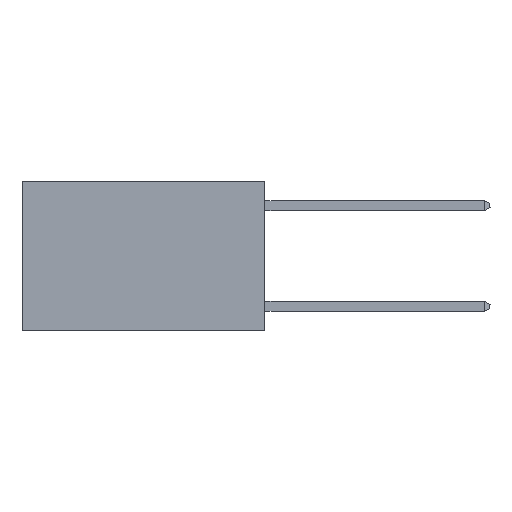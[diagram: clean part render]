
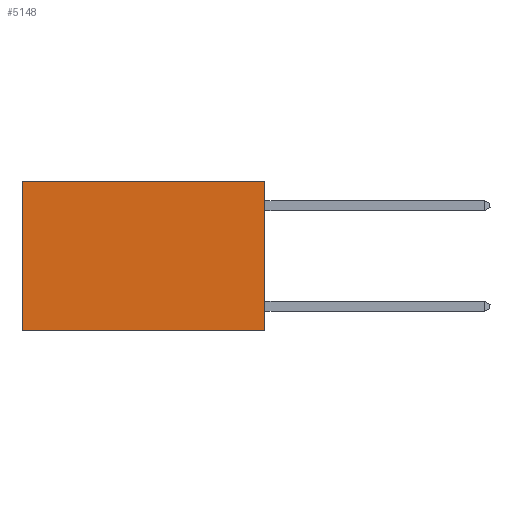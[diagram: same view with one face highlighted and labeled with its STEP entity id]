
A CAD part, left-side view. The second image highlights one B-rep face of the part: STEP entity #5148.
In plain terms, the highlighted planar face has unit normal (-1, 0, 0).
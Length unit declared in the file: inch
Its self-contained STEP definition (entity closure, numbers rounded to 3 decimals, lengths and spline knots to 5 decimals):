
#592 = VERTEX_POINT ( 'NONE', #12419 ) ;
#598 = CARTESIAN_POINT ( 'NONE',  ( 0.2625, 0., 0. ) ) ;
#2513 = ORIENTED_EDGE ( 'NONE', *, *, #7910, .F. ) ;
#3493 = VECTOR ( 'NONE', #13139, 39.37008 ) ;
#5148 = ADVANCED_FACE ( 'NONE', ( #5627 ), #16722, .F. ) ;
#5163 = ORIENTED_EDGE ( 'NONE', *, *, #24002, .T. ) ;
#5627 = FACE_OUTER_BOUND ( 'NONE', #24425, .T. ) ;
#6608 = VECTOR ( 'NONE', #28049, 39.37008 ) ;
#7044 = VERTEX_POINT ( 'NONE', #598 ) ;
#7422 = CARTESIAN_POINT ( 'NONE',  ( 0.2625, 0.6, 0. ) ) ;
#7807 = CARTESIAN_POINT ( 'NONE',  ( 0.2625, 0.6, -0.37 ) ) ;
#7910 = EDGE_CURVE ( 'NONE', #7044, #592, #19146, .T. ) ;
#8256 = DIRECTION ( 'NONE',  ( 1., 0., 0. ) ) ;
#9768 = LINE ( 'NONE', #16465, #15354 ) ;
#10593 = EDGE_CURVE ( 'NONE', #592, #24488, #26224, .T. ) ;
#12419 = CARTESIAN_POINT ( 'NONE',  ( 0.2625, 0., -0.37 ) ) ;
#13139 = DIRECTION ( 'NONE',  ( 0., 1., 0. ) ) ;
#15354 = VECTOR ( 'NONE', #27474, 39.37008 ) ;
#15512 = CARTESIAN_POINT ( 'NONE',  ( 0.2625, 0., -0.37 ) ) ;
#15884 = CARTESIAN_POINT ( 'NONE',  ( 0.2625, 0.6, 0. ) ) ;
#16465 = CARTESIAN_POINT ( 'NONE',  ( 0.2625, 0., 0. ) ) ;
#16722 = PLANE ( 'NONE',  #17514 ) ;
#17030 = EDGE_CURVE ( 'NONE', #28348, #24488, #18834, .T. ) ;
#17514 = AXIS2_PLACEMENT_3D ( 'NONE', #23709, #8256, #19095 ) ;
#18834 = LINE ( 'NONE', #7422, #6608 ) ;
#19095 = DIRECTION ( 'NONE',  ( 0., 0., -1. ) ) ;
#19146 = LINE ( 'NONE', #21529, #24289 ) ;
#21231 = DIRECTION ( 'NONE',  ( 0., 0., -1. ) ) ;
#21529 = CARTESIAN_POINT ( 'NONE',  ( 0.2625, 0., 0. ) ) ;
#23230 = ORIENTED_EDGE ( 'NONE', *, *, #17030, .T. ) ;
#23709 = CARTESIAN_POINT ( 'NONE',  ( 0.2625, 0., 0. ) ) ;
#24002 = EDGE_CURVE ( 'NONE', #7044, #28348, #9768, .T. ) ;
#24266 = ORIENTED_EDGE ( 'NONE', *, *, #10593, .F. ) ;
#24289 = VECTOR ( 'NONE', #21231, 39.37008 ) ;
#24425 = EDGE_LOOP ( 'NONE', ( #23230, #24266, #2513, #5163 ) ) ;
#24488 = VERTEX_POINT ( 'NONE', #7807 ) ;
#26224 = LINE ( 'NONE', #15512, #3493 ) ;
#27474 = DIRECTION ( 'NONE',  ( 0., 1., 0. ) ) ;
#28049 = DIRECTION ( 'NONE',  ( 0., 0., -1. ) ) ;
#28348 = VERTEX_POINT ( 'NONE', #15884 ) ;
